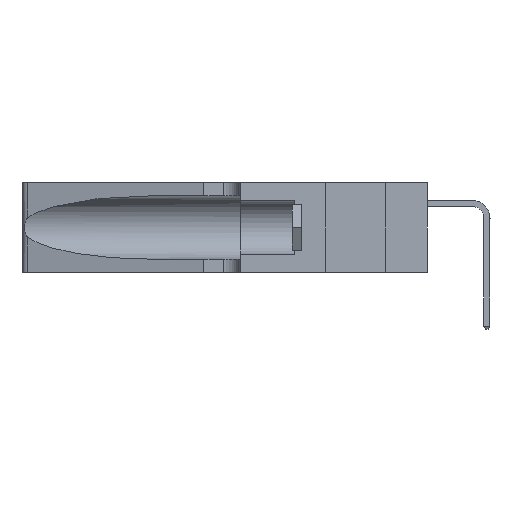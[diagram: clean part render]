
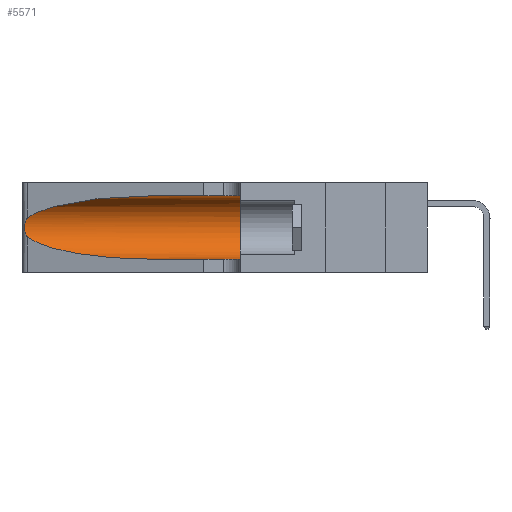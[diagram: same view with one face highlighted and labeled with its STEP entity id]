
A CAD part, left-side view. The second image highlights one B-rep face of the part: STEP entity #5571.
In plain terms, the highlighted cylindrical face has radius 3.308 mm (diameter 6.617 mm), a partial arc.
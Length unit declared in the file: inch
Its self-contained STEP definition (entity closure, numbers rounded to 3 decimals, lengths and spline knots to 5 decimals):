
#333 = LINE ( 'NONE', #26563, #43201 ) ;
#1729 = EDGE_CURVE ( 'NONE', #33002, #22678, #26634, .T. ) ;
#2538 = CARTESIAN_POINT ( 'NONE',  ( 0.26018, 1.23835, 0.19895 ) ) ;
#2868 = CARTESIAN_POINT ( 'NONE',  ( 0.1305, 0.35, 0.185 ) ) ;
#3090 = VERTEX_POINT ( 'NONE', #28936 ) ;
#3785 = VERTEX_POINT ( 'NONE', #25637 ) ;
#5168 = CARTESIAN_POINT ( 'NONE',  ( 0.1305, 0.35, 0.05475 ) ) ;
#5218 = CARTESIAN_POINT ( 'NONE',  ( 0.2373, 1.15595, 0.08982 ) ) ;
#5571 = ADVANCED_FACE ( 'NONE', ( #42336 ), #41300, .F. ) ;
#5937 = CARTESIAN_POINT ( 'NONE',  ( 0.26075, 1.23896, 0.178 ) ) ;
#6258 = DIRECTION ( 'NONE',  ( 0., 0., 1. ) ) ;
#8620 = CARTESIAN_POINT ( 'NONE',  ( 0.18966, 0.96281, 0.05475 ) ) ;
#9341 = CARTESIAN_POINT ( 'NONE',  ( 0.25856, 1.23593, 0.16098 ) ) ;
#10175 = CARTESIAN_POINT ( 'NONE',  ( 0.1305, 0.72297, 0.05475 ) ) ;
#10248 = CARTESIAN_POINT ( 'NONE',  ( 0.1305, 0.35, 0.31525 ) ) ;
#10722 = EDGE_CURVE ( 'NONE', #25702, #22678, #37739, .T. ) ;
#11271 = AXIS2_PLACEMENT_3D ( 'NONE', #2868, #26591, #6258 ) ;
#11587 = VERTEX_POINT ( 'NONE', #24167 ) ;
#12373 = CARTESIAN_POINT ( 'NONE',  ( 0.1305, 0.72297, 0.31525 ) ) ;
#12755 = CARTESIAN_POINT ( 'NONE',  ( 0.25639, 1.23186, 0.15144 ) ) ;
#13373 = EDGE_CURVE ( 'NONE', #3785, #3090, #33926, .T. ) ;
#14799 = DIRECTION ( 'NONE',  ( 0., 0., -1. ) ) ;
#15794 = CARTESIAN_POINT ( 'NONE',  ( 0.18966, 0.96281, 0.31525 ) ) ;
#15916 = EDGE_CURVE ( 'NONE', #3785, #33002, #333, .T. ) ;
#16189 = CARTESIAN_POINT ( 'NONE',  ( 0.25487, 1.22718, 0.14631 ) ) ;
#16479 = DIRECTION ( 'NONE',  ( 0., -1., 0. ) ) ;
#17265 =( BOUNDED_CURVE ( )  B_SPLINE_CURVE ( 3, ( #25547, #5218, #8620, #32352 ),
 .UNSPECIFIED., .F., .F. ) 
 B_SPLINE_CURVE_WITH_KNOTS ( ( 4, 4 ),
 ( 3.44316, 4.71239 ),
 .UNSPECIFIED. ) 
 CURVE ( )  GEOMETRIC_REPRESENTATION_ITEM ( )  RATIONAL_B_SPLINE_CURVE ( ( 1., 0.87, 0.87, 1. ) ) 
 REPRESENTATION_ITEM ( '' )  );
#17825 = B_SPLINE_CURVE_WITH_KNOTS ( 'NONE', 3,
 ( #36311, #39699, #19431, #43048, #22841, #2538, #26271, #5937, #29679, #9341, #33078, #12755, #36469, #16189 ),
 .UNSPECIFIED., .F., .F.,
 ( 4, 2, 2, 2, 2, 2, 4 ),
 ( 0., 0.00027, 0.00053, 0.00107, 0.0016, 0.00187, 0.00214 ),
 .UNSPECIFIED. ) ;
#18243 = ORIENTED_EDGE ( 'NONE', *, *, #29948, .T. ) ;
#19201 = CARTESIAN_POINT ( 'NONE',  ( 0.25487, 1.22718, 0.22369 ) ) ;
#19431 = CARTESIAN_POINT ( 'NONE',  ( 0.25639, 1.23184, 0.21858 ) ) ;
#19591 = CARTESIAN_POINT ( 'NONE',  ( 0.1305, 1.61858, 0.05475 ) ) ;
#22678 = VERTEX_POINT ( 'NONE', #5168 ) ;
#22733 = ORIENTED_EDGE ( 'NONE', *, *, #15916, .F. ) ;
#22841 = CARTESIAN_POINT ( 'NONE',  ( 0.25854, 1.2359, 0.20912 ) ) ;
#24167 = CARTESIAN_POINT ( 'NONE',  ( 0.25487, 1.22718, 0.14631 ) ) ;
#24557 = ORIENTED_EDGE ( 'NONE', *, *, #1729, .F. ) ;
#25547 = CARTESIAN_POINT ( 'NONE',  ( 0.25487, 1.22718, 0.14631 ) ) ;
#25637 = CARTESIAN_POINT ( 'NONE',  ( 0.1305, 0.72297, 0.31525 ) ) ;
#25702 = VERTEX_POINT ( 'NONE', #10175 ) ;
#26271 = CARTESIAN_POINT ( 'NONE',  ( 0.26075, 1.23896, 0.19203 ) ) ;
#26563 = CARTESIAN_POINT ( 'NONE',  ( 0.1305, 1.61858, 0.31525 ) ) ;
#26591 = DIRECTION ( 'NONE',  ( 0., 1., 0. ) ) ;
#26634 = CIRCLE ( 'NONE', #11271, 0.13025 ) ;
#26739 = ORIENTED_EDGE ( 'NONE', *, *, #13373, .T. ) ;
#28936 = CARTESIAN_POINT ( 'NONE',  ( 0.25487, 1.22718, 0.22369 ) ) ;
#29679 = CARTESIAN_POINT ( 'NONE',  ( 0.26017, 1.23833, 0.17102 ) ) ;
#29948 = EDGE_CURVE ( 'NONE', #3090, #11587, #17825, .T. ) ;
#31696 = CARTESIAN_POINT ( 'NONE',  ( 0.1305, 1.61858, 0.185 ) ) ;
#32352 = CARTESIAN_POINT ( 'NONE',  ( 0.1305, 0.72297, 0.05475 ) ) ;
#33002 = VERTEX_POINT ( 'NONE', #10248 ) ;
#33078 = CARTESIAN_POINT ( 'NONE',  ( 0.25789, 1.23486, 0.15765 ) ) ;
#33926 =( BOUNDED_CURVE ( )  B_SPLINE_CURVE ( 3, ( #12373, #15794, #39463, #19201 ),
 .UNSPECIFIED., .F., .T. ) 
 B_SPLINE_CURVE_WITH_KNOTS ( ( 4, 4 ),
 ( 1.5708, 2.84003 ),
 .UNSPECIFIED. ) 
 CURVE ( )  GEOMETRIC_REPRESENTATION_ITEM ( )  RATIONAL_B_SPLINE_CURVE ( ( 1., 0.87, 0.87, 1. ) ) 
 REPRESENTATION_ITEM ( '' )  );
#36311 = CARTESIAN_POINT ( 'NONE',  ( 0.25487, 1.22718, 0.22369 ) ) ;
#36469 = CARTESIAN_POINT ( 'NONE',  ( 0.25555, 1.22993, 0.14849 ) ) ;
#36678 = VECTOR ( 'NONE', #39999, 39.37008 ) ;
#37739 = LINE ( 'NONE', #19591, #36678 ) ;
#38095 = AXIS2_PLACEMENT_3D ( 'NONE', #31696, #41831, #14799 ) ;
#38357 = ORIENTED_EDGE ( 'NONE', *, *, #10722, .T. ) ;
#39463 = CARTESIAN_POINT ( 'NONE',  ( 0.2373, 1.15595, 0.28018 ) ) ;
#39699 = CARTESIAN_POINT ( 'NONE',  ( 0.25555, 1.22994, 0.2215 ) ) ;
#39999 = DIRECTION ( 'NONE',  ( 0., -1., 0. ) ) ;
#41300 = CYLINDRICAL_SURFACE ( 'NONE', #38095, 0.13025 ) ;
#41831 = DIRECTION ( 'NONE',  ( 0., -1., 0. ) ) ;
#42133 = EDGE_LOOP ( 'NONE', ( #26739, #18243, #42935, #38357, #24557, #22733 ) ) ;
#42336 = FACE_OUTER_BOUND ( 'NONE', #42133, .T. ) ;
#42342 = EDGE_CURVE ( 'NONE', #11587, #25702, #17265, .T. ) ;
#42935 = ORIENTED_EDGE ( 'NONE', *, *, #42342, .T. ) ;
#43048 = CARTESIAN_POINT ( 'NONE',  ( 0.25787, 1.23484, 0.2124 ) ) ;
#43201 = VECTOR ( 'NONE', #16479, 39.37008 ) ;
